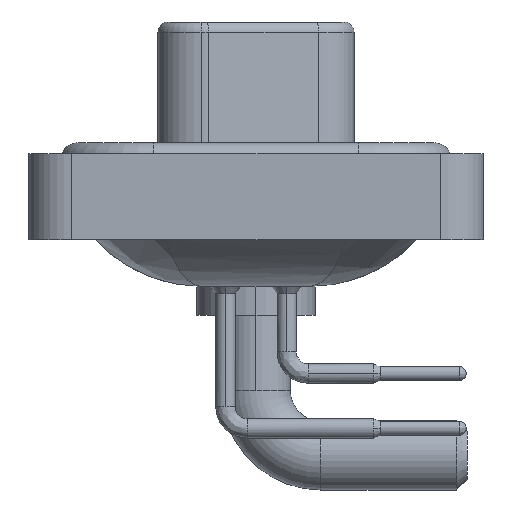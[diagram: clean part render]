
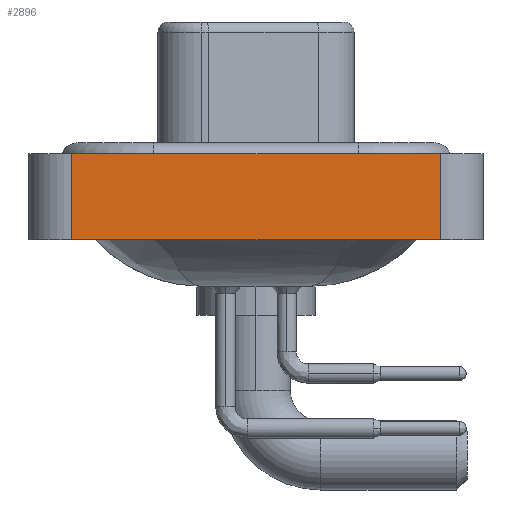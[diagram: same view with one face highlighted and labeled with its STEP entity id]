
A CAD part, left-side view. The second image highlights one B-rep face of the part: STEP entity #2896.
In plain terms, the highlighted planar face has unit normal (-1, 0, 0).
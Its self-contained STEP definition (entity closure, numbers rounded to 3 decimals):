
#486 = EDGE_CURVE ( 'NONE', #2296, #960, #8290, .T. ) ;
#960 = VERTEX_POINT ( 'NONE', #17183 ) ;
#1346 = FACE_OUTER_BOUND ( 'NONE', #9244, .T. ) ;
#2197 = CARTESIAN_POINT ( 'NONE',  ( -7.25, 8.55, -3.6 ) ) ;
#2258 = CARTESIAN_POINT ( 'NONE',  ( -7.25, -8.55, 0.4 ) ) ;
#2296 = VERTEX_POINT ( 'NONE', #2197 ) ;
#2546 = CARTESIAN_POINT ( 'NONE',  ( -7.25, -8.55, -3.6 ) ) ;
#2658 = DIRECTION ( 'NONE',  ( 0., 0., 1. ) ) ;
#2896 = ADVANCED_FACE ( 'NONE', ( #1346 ), #9895, .T. ) ;
#3829 = ORIENTED_EDGE ( 'NONE', *, *, #20240, .F. ) ;
#4941 = DIRECTION ( 'NONE',  ( 0., -1., 0. ) ) ;
#5407 = AXIS2_PLACEMENT_3D ( 'NONE', #8142, #8380, #11637 ) ;
#8142 = CARTESIAN_POINT ( 'NONE',  ( -7.25, -8.55, -3.6 ) ) ;
#8290 = LINE ( 'NONE', #13857, #16298 ) ;
#8380 = DIRECTION ( 'NONE',  ( -1., 0., 0. ) ) ;
#8497 = CARTESIAN_POINT ( 'NONE',  ( -7.25, -8.55, 0.4 ) ) ;
#9244 = EDGE_LOOP ( 'NONE', ( #9613, #20764, #3829, #22319 ) ) ;
#9296 = DIRECTION ( 'NONE',  ( 0., -1., 0. ) ) ;
#9613 = ORIENTED_EDGE ( 'NONE', *, *, #11545, .T. ) ;
#9895 = PLANE ( 'NONE',  #5407 ) ;
#11156 = VECTOR ( 'NONE', #2658, 1000. ) ;
#11545 = EDGE_CURVE ( 'NONE', #960, #22128, #20000, .T. ) ;
#11637 = DIRECTION ( 'NONE',  ( 0., 0., 1. ) ) ;
#12282 = CARTESIAN_POINT ( 'NONE',  ( -7.25, 8.55, 0.4 ) ) ;
#12406 = VECTOR ( 'NONE', #9296, 1000. ) ;
#12799 = VERTEX_POINT ( 'NONE', #12282 ) ;
#13657 = CARTESIAN_POINT ( 'NONE',  ( -7.25, 8.55, -3.6 ) ) ;
#13857 = CARTESIAN_POINT ( 'NONE',  ( -7.25, -8.55, -3.6 ) ) ;
#13888 = DIRECTION ( 'NONE',  ( 0., 0., 1. ) ) ;
#16298 = VECTOR ( 'NONE', #4941, 1000. ) ;
#17183 = CARTESIAN_POINT ( 'NONE',  ( -7.25, -8.55, -3.6 ) ) ;
#18092 = LINE ( 'NONE', #2258, #12406 ) ;
#20000 = LINE ( 'NONE', #2546, #11156 ) ;
#20240 = EDGE_CURVE ( 'NONE', #2296, #12799, #22756, .T. ) ;
#20764 = ORIENTED_EDGE ( 'NONE', *, *, #21221, .F. ) ;
#21221 = EDGE_CURVE ( 'NONE', #12799, #22128, #18092, .T. ) ;
#22128 = VERTEX_POINT ( 'NONE', #8497 ) ;
#22306 = VECTOR ( 'NONE', #13888, 1000. ) ;
#22319 = ORIENTED_EDGE ( 'NONE', *, *, #486, .T. ) ;
#22756 = LINE ( 'NONE', #13657, #22306 ) ;
